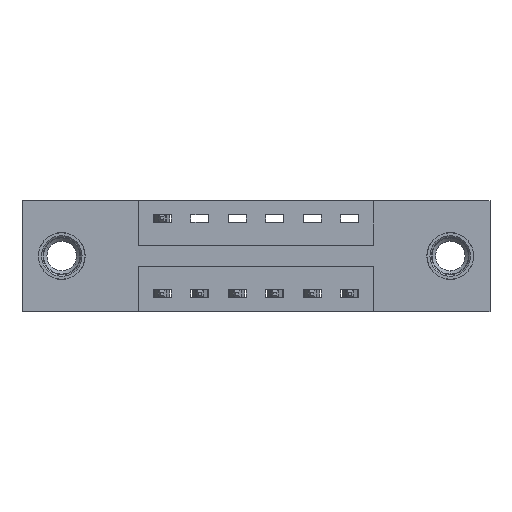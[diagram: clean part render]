
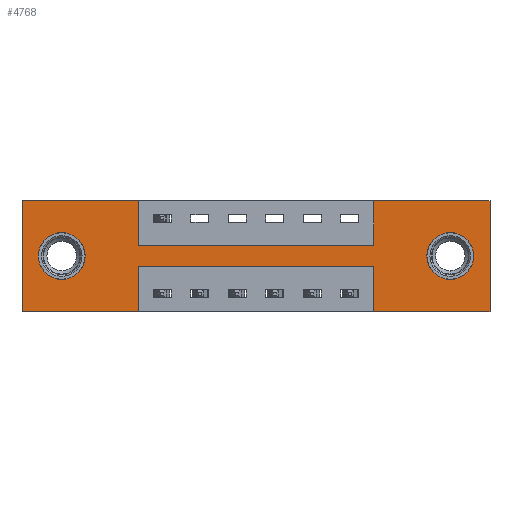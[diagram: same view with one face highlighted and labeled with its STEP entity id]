
A CAD part, front view. The second image highlights one B-rep face of the part: STEP entity #4768.
In plain terms, the highlighted planar face has unit normal (0, -1, 0).
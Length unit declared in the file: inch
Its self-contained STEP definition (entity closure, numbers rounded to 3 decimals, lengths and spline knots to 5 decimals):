
#29 = EDGE_CURVE ( 'NONE', #1184, #4798, #1197, .T. ) ;
#102 = DIRECTION ( 'NONE',  ( 0., 0., 1. ) ) ;
#107 = CARTESIAN_POINT ( 'NONE',  ( 1.1725, 0., 0. ) ) ;
#306 = AXIS2_PLACEMENT_3D ( 'NONE', #4405, #9696, #5152 ) ;
#317 = LINE ( 'NONE', #8979, #4105 ) ;
#390 = EDGE_LOOP ( 'NONE', ( #746, #6995 ) ) ;
#405 = DIRECTION ( 'NONE',  ( 0., 1., 0. ) ) ;
#549 = LINE ( 'NONE', #4893, #8343 ) ;
#580 = VERTEX_POINT ( 'NONE', #4412 ) ;
#654 = VERTEX_POINT ( 'NONE', #4539 ) ;
#746 = ORIENTED_EDGE ( 'NONE', *, *, #9372, .T. ) ;
#759 = EDGE_CURVE ( 'NONE', #5077, #6816, #8839, .T. ) ;
#766 = PLANE ( 'NONE',  #7162 ) ;
#801 = LINE ( 'NONE', #5071, #8823 ) ;
#859 = EDGE_CURVE ( 'NONE', #7631, #9138, #9654, .T. ) ;
#1069 = EDGE_CURVE ( 'NONE', #8629, #7341, #2452, .T. ) ;
#1077 = EDGE_CURVE ( 'NONE', #3575, #3677, #6214, .T. ) ;
#1184 = VERTEX_POINT ( 'NONE', #2308 ) ;
#1197 = LINE ( 'NONE', #3797, #5433 ) ;
#1239 = EDGE_LOOP ( 'NONE', ( #9492, #5107, #4999, #3487, #2680, #7388, #1277, #8714, #7856, #3174, #5563, #2357 ) ) ;
#1277 = ORIENTED_EDGE ( 'NONE', *, *, #6697, .F. ) ;
#1294 = VERTEX_POINT ( 'NONE', #7692 ) ;
#1295 = LINE ( 'NONE', #3233, #3315 ) ;
#1405 = DIRECTION ( 'NONE',  ( 1., 0., 0. ) ) ;
#1576 = CARTESIAN_POINT ( 'NONE',  ( 0.3875, 0., -0.15 ) ) ;
#1602 = CARTESIAN_POINT ( 'NONE',  ( 0.1325, 0., -0.185 ) ) ;
#1641 = AXIS2_PLACEMENT_3D ( 'NONE', #1832, #7099, #2596 ) ;
#1648 = CIRCLE ( 'NONE', #1641, 0.078 ) ;
#1743 = VERTEX_POINT ( 'NONE', #8247 ) ;
#1765 = CARTESIAN_POINT ( 'NONE',  ( 1.1725, 0., -0.15 ) ) ;
#1779 = CARTESIAN_POINT ( 'NONE',  ( 1.56, 0., 0. ) ) ;
#1788 = CARTESIAN_POINT ( 'NONE',  ( 0., 0., -0.37 ) ) ;
#1832 = CARTESIAN_POINT ( 'NONE',  ( 0.1325, 0., -0.185 ) ) ;
#2000 = CIRCLE ( 'NONE', #6228, 0.078 ) ;
#2212 = VECTOR ( 'NONE', #1405, 39.37008 ) ;
#2308 = CARTESIAN_POINT ( 'NONE',  ( 0.3875, 0., 0. ) ) ;
#2335 = CARTESIAN_POINT ( 'NONE',  ( 0.3875, 0., -0.37 ) ) ;
#2357 = ORIENTED_EDGE ( 'NONE', *, *, #4954, .F. ) ;
#2368 = DIRECTION ( 'NONE',  ( 0., 0., 1. ) ) ;
#2384 = AXIS2_PLACEMENT_3D ( 'NONE', #4912, #405, #5687 ) ;
#2452 = CIRCLE ( 'NONE', #306, 0.078 ) ;
#2491 = FACE_BOUND ( 'NONE', #390, .T. ) ;
#2596 = DIRECTION ( 'NONE',  ( 0., 0., 1. ) ) ;
#2603 = CARTESIAN_POINT ( 'NONE',  ( 0.3875, 0., -0.22 ) ) ;
#2680 = ORIENTED_EDGE ( 'NONE', *, *, #6608, .F. ) ;
#2832 = LINE ( 'NONE', #1788, #8838 ) ;
#3031 = DIRECTION ( 'NONE',  ( 0., 0., 1. ) ) ;
#3078 = CARTESIAN_POINT ( 'NONE',  ( 0.3875, 0., -0.15 ) ) ;
#3174 = ORIENTED_EDGE ( 'NONE', *, *, #5617, .F. ) ;
#3233 = CARTESIAN_POINT ( 'NONE',  ( 0., 0., 0. ) ) ;
#3315 = VECTOR ( 'NONE', #7729, 39.37008 ) ;
#3352 = ORIENTED_EDGE ( 'NONE', *, *, #5822, .T. ) ;
#3431 = DIRECTION ( 'NONE',  ( -1., 0., 0. ) ) ;
#3487 = ORIENTED_EDGE ( 'NONE', *, *, #759, .F. ) ;
#3575 = VERTEX_POINT ( 'NONE', #107 ) ;
#3677 = VERTEX_POINT ( 'NONE', #1779 ) ;
#3796 = DIRECTION ( 'NONE',  ( 0., -1., 0. ) ) ;
#3797 = CARTESIAN_POINT ( 'NONE',  ( 0.3875, 0., 0. ) ) ;
#3836 = DIRECTION ( 'NONE',  ( 1., 0., 0. ) ) ;
#3978 = CARTESIAN_POINT ( 'NONE',  ( 1.4275, 0., -0.263 ) ) ;
#4105 = VECTOR ( 'NONE', #9750, 39.37008 ) ;
#4246 = CARTESIAN_POINT ( 'NONE',  ( 1.56, 0., -0.37 ) ) ;
#4405 = CARTESIAN_POINT ( 'NONE',  ( 1.4275, 0., -0.185 ) ) ;
#4412 = CARTESIAN_POINT ( 'NONE',  ( 0.1325, 0., -0.107 ) ) ;
#4461 = CARTESIAN_POINT ( 'NONE',  ( 0., 0., -0.37 ) ) ;
#4473 = CARTESIAN_POINT ( 'NONE',  ( 1.4275, 0., -0.107 ) ) ;
#4539 = CARTESIAN_POINT ( 'NONE',  ( 0., 0., 0. ) ) ;
#4670 = CARTESIAN_POINT ( 'NONE',  ( 0., 0., -0.37 ) ) ;
#4768 = ADVANCED_FACE ( 'NONE', ( #6496, #2491, #4929 ), #766, .T. ) ;
#4798 = VERTEX_POINT ( 'NONE', #3078 ) ;
#4816 = VECTOR ( 'NONE', #6916, 39.37008 ) ;
#4893 = CARTESIAN_POINT ( 'NONE',  ( 0.3875, 0., -0.22 ) ) ;
#4912 = CARTESIAN_POINT ( 'NONE',  ( 1.4275, 0., -0.185 ) ) ;
#4929 = FACE_OUTER_BOUND ( 'NONE', #1239, .T. ) ;
#4954 = EDGE_CURVE ( 'NONE', #9138, #6058, #2832, .T. ) ;
#4999 = ORIENTED_EDGE ( 'NONE', *, *, #5437, .F. ) ;
#5071 = CARTESIAN_POINT ( 'NONE',  ( 1.56, 0., 0. ) ) ;
#5077 = VERTEX_POINT ( 'NONE', #4246 ) ;
#5089 = LINE ( 'NONE', #8403, #6408 ) ;
#5107 = ORIENTED_EDGE ( 'NONE', *, *, #7069, .F. ) ;
#5152 = DIRECTION ( 'NONE',  ( 0., 0., -1. ) ) ;
#5433 = VECTOR ( 'NONE', #9082, 39.37008 ) ;
#5437 = EDGE_CURVE ( 'NONE', #6816, #1294, #8359, .T. ) ;
#5563 = ORIENTED_EDGE ( 'NONE', *, *, #7471, .F. ) ;
#5617 = EDGE_CURVE ( 'NONE', #654, #1184, #1295, .T. ) ;
#5687 = DIRECTION ( 'NONE',  ( 0., 0., -1. ) ) ;
#5822 = EDGE_CURVE ( 'NONE', #7341, #8629, #9681, .T. ) ;
#6058 = VERTEX_POINT ( 'NONE', #4461 ) ;
#6152 = EDGE_CURVE ( 'NONE', #1743, #580, #2000, .T. ) ;
#6214 = LINE ( 'NONE', #6699, #2212 ) ;
#6228 = AXIS2_PLACEMENT_3D ( 'NONE', #1602, #6875, #2368 ) ;
#6362 = VECTOR ( 'NONE', #3031, 39.37008 ) ;
#6408 = VECTOR ( 'NONE', #102, 39.37008 ) ;
#6496 = FACE_BOUND ( 'NONE', #6984, .T. ) ;
#6608 = EDGE_CURVE ( 'NONE', #3677, #5077, #801, .T. ) ;
#6697 = EDGE_CURVE ( 'NONE', #9344, #3575, #317, .T. ) ;
#6699 = CARTESIAN_POINT ( 'NONE',  ( 0., 0., 0. ) ) ;
#6816 = VERTEX_POINT ( 'NONE', #9107 ) ;
#6875 = DIRECTION ( 'NONE',  ( 0., 1., 0. ) ) ;
#6916 = DIRECTION ( 'NONE',  ( -1., 0., 0. ) ) ;
#6984 = EDGE_LOOP ( 'NONE', ( #3352, #8049 ) ) ;
#6995 = ORIENTED_EDGE ( 'NONE', *, *, #6152, .T. ) ;
#7069 = EDGE_CURVE ( 'NONE', #1294, #7631, #549, .T. ) ;
#7076 = DIRECTION ( 'NONE',  ( 0., 0., -1. ) ) ;
#7099 = DIRECTION ( 'NONE',  ( 0., 1., 0. ) ) ;
#7162 = AXIS2_PLACEMENT_3D ( 'NONE', #7542, #3796, #9079 ) ;
#7341 = VERTEX_POINT ( 'NONE', #4473 ) ;
#7344 = DIRECTION ( 'NONE',  ( 0., 0., -1. ) ) ;
#7388 = ORIENTED_EDGE ( 'NONE', *, *, #1077, .F. ) ;
#7471 = EDGE_CURVE ( 'NONE', #6058, #654, #5089, .T. ) ;
#7542 = CARTESIAN_POINT ( 'NONE',  ( 0., 0., -0.37 ) ) ;
#7617 = VECTOR ( 'NONE', #7076, 39.37008 ) ;
#7631 = VERTEX_POINT ( 'NONE', #2603 ) ;
#7692 = CARTESIAN_POINT ( 'NONE',  ( 1.1725, 0., -0.22 ) ) ;
#7729 = DIRECTION ( 'NONE',  ( 1., 0., 0. ) ) ;
#7742 = DIRECTION ( 'NONE',  ( -1., 0., 0. ) ) ;
#7856 = ORIENTED_EDGE ( 'NONE', *, *, #29, .F. ) ;
#7956 = EDGE_CURVE ( 'NONE', #4798, #9344, #8398, .T. ) ;
#8049 = ORIENTED_EDGE ( 'NONE', *, *, #1069, .T. ) ;
#8147 = VECTOR ( 'NONE', #3836, 39.37008 ) ;
#8247 = CARTESIAN_POINT ( 'NONE',  ( 0.1325, 0., -0.263 ) ) ;
#8301 = CARTESIAN_POINT ( 'NONE',  ( 1.1725, 0., -0.37 ) ) ;
#8343 = VECTOR ( 'NONE', #3431, 39.37008 ) ;
#8359 = LINE ( 'NONE', #8301, #6362 ) ;
#8398 = LINE ( 'NONE', #1576, #8147 ) ;
#8403 = CARTESIAN_POINT ( 'NONE',  ( 0., 0., 0. ) ) ;
#8629 = VERTEX_POINT ( 'NONE', #3978 ) ;
#8714 = ORIENTED_EDGE ( 'NONE', *, *, #7956, .F. ) ;
#8823 = VECTOR ( 'NONE', #7344, 39.37008 ) ;
#8838 = VECTOR ( 'NONE', #7742, 39.37008 ) ;
#8839 = LINE ( 'NONE', #4670, #4816 ) ;
#8979 = CARTESIAN_POINT ( 'NONE',  ( 1.1725, 0., 0. ) ) ;
#9079 = DIRECTION ( 'NONE',  ( 0., 0., -1. ) ) ;
#9082 = DIRECTION ( 'NONE',  ( 0., 0., -1. ) ) ;
#9107 = CARTESIAN_POINT ( 'NONE',  ( 1.1725, 0., -0.37 ) ) ;
#9138 = VERTEX_POINT ( 'NONE', #2335 ) ;
#9329 = CARTESIAN_POINT ( 'NONE',  ( 0.3875, 0., -0.37 ) ) ;
#9344 = VERTEX_POINT ( 'NONE', #1765 ) ;
#9372 = EDGE_CURVE ( 'NONE', #580, #1743, #1648, .T. ) ;
#9492 = ORIENTED_EDGE ( 'NONE', *, *, #859, .F. ) ;
#9654 = LINE ( 'NONE', #9329, #7617 ) ;
#9681 = CIRCLE ( 'NONE', #2384, 0.078 ) ;
#9696 = DIRECTION ( 'NONE',  ( 0., 1., 0. ) ) ;
#9750 = DIRECTION ( 'NONE',  ( 0., 0., 1. ) ) ;
